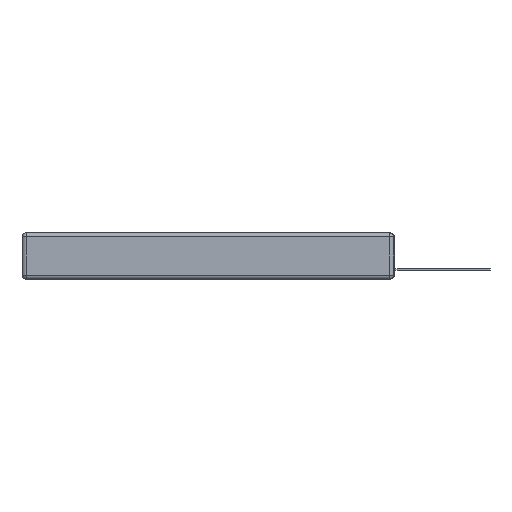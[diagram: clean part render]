
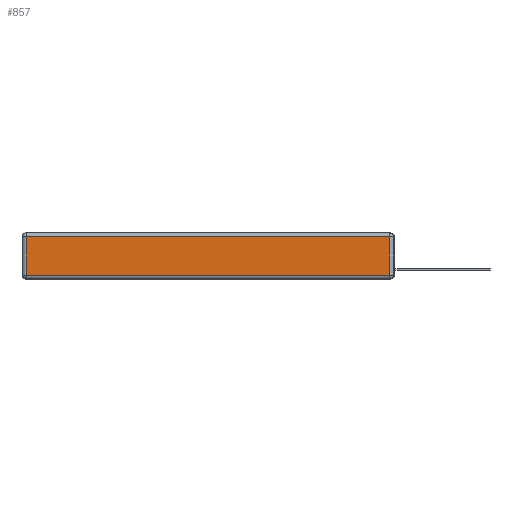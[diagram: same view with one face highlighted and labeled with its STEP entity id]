
A CAD part, left-side view. The second image highlights one B-rep face of the part: STEP entity #857.
In plain terms, the highlighted planar face has unit normal (-1, 0, 0).
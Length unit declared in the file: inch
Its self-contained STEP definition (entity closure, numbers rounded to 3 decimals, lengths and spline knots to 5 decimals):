
#857 = ADVANCED_FACE ( 'NONE', ( #25776 ), #2078, .T. ) ;
#1363 = VERTEX_POINT ( 'NONE', #4417 ) ;
#2078 = PLANE ( 'NONE',  #13044 ) ;
#2579 = EDGE_CURVE ( 'NONE', #10177, #7209, #17652, .T. ) ;
#3431 = VERTEX_POINT ( 'NONE', #16480 ) ;
#3548 = DIRECTION ( 'NONE',  ( 0., 1., 0. ) ) ;
#4378 = ORIENTED_EDGE ( 'NONE', *, *, #15978, .T. ) ;
#4417 = CARTESIAN_POINT ( 'NONE',  ( 0., 2.72, -0.03 ) ) ;
#5298 = DIRECTION ( 'NONE',  ( -1., 0., 0. ) ) ;
#5773 = ORIENTED_EDGE ( 'NONE', *, *, #2579, .T. ) ;
#6669 = CARTESIAN_POINT ( 'NONE',  ( 0., 0.03, -0.03 ) ) ;
#6741 = DIRECTION ( 'NONE',  ( 0., -1., 0. ) ) ;
#7209 = VERTEX_POINT ( 'NONE', #6669 ) ;
#7560 = CARTESIAN_POINT ( 'NONE',  ( 0., 0., -0.343 ) ) ;
#7674 = CARTESIAN_POINT ( 'NONE',  ( 0., 0.03, -0.343 ) ) ;
#8061 = LINE ( 'NONE', #12164, #19949 ) ;
#10139 = EDGE_CURVE ( 'NONE', #1363, #3431, #20645, .T. ) ;
#10177 = VERTEX_POINT ( 'NONE', #22665 ) ;
#10591 = CARTESIAN_POINT ( 'NONE',  ( 0., 0., -0.313 ) ) ;
#12164 = CARTESIAN_POINT ( 'NONE',  ( 0., 2.75, -0.03 ) ) ;
#13025 = VECTOR ( 'NONE', #6741, 39.37008 ) ;
#13044 = AXIS2_PLACEMENT_3D ( 'NONE', #7560, #5298, #15671 ) ;
#13777 = EDGE_LOOP ( 'NONE', ( #4378, #5773, #23849, #22865 ) ) ;
#15671 = DIRECTION ( 'NONE',  ( 0., 0., 1. ) ) ;
#15978 = EDGE_CURVE ( 'NONE', #3431, #10177, #21091, .T. ) ;
#16480 = CARTESIAN_POINT ( 'NONE',  ( 0., 2.72, -0.313 ) ) ;
#17652 = LINE ( 'NONE', #7674, #19322 ) ;
#18279 = CARTESIAN_POINT ( 'NONE',  ( 0., 2.72, -0.343 ) ) ;
#19322 = VECTOR ( 'NONE', #25756, 39.37008 ) ;
#19855 = VECTOR ( 'NONE', #22246, 39.37008 ) ;
#19949 = VECTOR ( 'NONE', #3548, 39.37008 ) ;
#20645 = LINE ( 'NONE', #18279, #19855 ) ;
#21091 = LINE ( 'NONE', #10591, #13025 ) ;
#22246 = DIRECTION ( 'NONE',  ( 0., 0., -1. ) ) ;
#22665 = CARTESIAN_POINT ( 'NONE',  ( 0., 0.03, -0.313 ) ) ;
#22865 = ORIENTED_EDGE ( 'NONE', *, *, #10139, .T. ) ;
#23849 = ORIENTED_EDGE ( 'NONE', *, *, #24168, .T. ) ;
#24168 = EDGE_CURVE ( 'NONE', #7209, #1363, #8061, .T. ) ;
#25756 = DIRECTION ( 'NONE',  ( 0., 0., 1. ) ) ;
#25776 = FACE_OUTER_BOUND ( 'NONE', #13777, .T. ) ;
